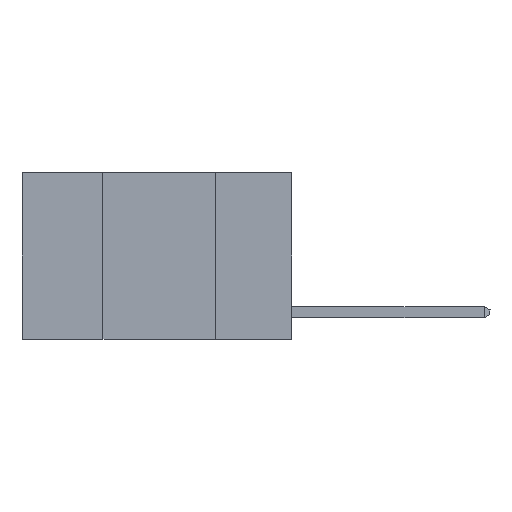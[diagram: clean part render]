
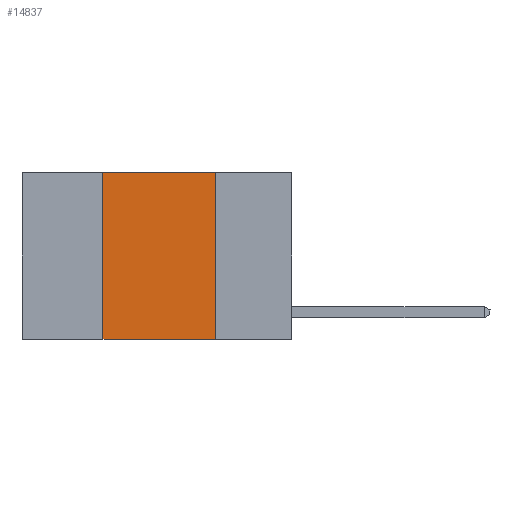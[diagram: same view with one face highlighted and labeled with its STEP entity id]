
A CAD part, left-side view. The second image highlights one B-rep face of the part: STEP entity #14837.
In plain terms, the highlighted planar face has unit normal (-1, 0, 0).
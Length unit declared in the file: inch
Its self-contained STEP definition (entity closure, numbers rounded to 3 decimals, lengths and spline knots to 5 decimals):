
#48 = CARTESIAN_POINT ( 'NONE',  ( 0., 0.42, 0. ) ) ;
#81 = ORIENTED_EDGE ( 'NONE', *, *, #13003, .F. ) ;
#543 = VECTOR ( 'NONE', #5132, 39.37008 ) ;
#2588 = DIRECTION ( 'NONE',  ( 0., -1., 0. ) ) ;
#3650 = DIRECTION ( 'NONE',  ( 0., 0., 1. ) ) ;
#3873 = ORIENTED_EDGE ( 'NONE', *, *, #11862, .F. ) ;
#3981 = CARTESIAN_POINT ( 'NONE',  ( 0., 0.6, 0. ) ) ;
#4129 = CARTESIAN_POINT ( 'NONE',  ( 0., 0.17, -0.37 ) ) ;
#4639 = ORIENTED_EDGE ( 'NONE', *, *, #11732, .T. ) ;
#4916 = PLANE ( 'NONE',  #13979 ) ;
#5132 = DIRECTION ( 'NONE',  ( 0., -1., 0. ) ) ;
#5195 = CARTESIAN_POINT ( 'NONE',  ( 0., 0.17, 0. ) ) ;
#6802 = DIRECTION ( 'NONE',  ( 1., 0., 0. ) ) ;
#6878 = VECTOR ( 'NONE', #3650, 39.37008 ) ;
#7377 = VERTEX_POINT ( 'NONE', #5195 ) ;
#7499 = LINE ( 'NONE', #16522, #9215 ) ;
#8285 = DIRECTION ( 'NONE',  ( 0., 0., -1. ) ) ;
#9215 = VECTOR ( 'NONE', #2588, 39.37008 ) ;
#11022 = DIRECTION ( 'NONE',  ( 0., 0., -1. ) ) ;
#11118 = ORIENTED_EDGE ( 'NONE', *, *, #17581, .F. ) ;
#11295 = LINE ( 'NONE', #12270, #12367 ) ;
#11732 = EDGE_CURVE ( 'NONE', #17272, #11993, #13965, .T. ) ;
#11862 = EDGE_CURVE ( 'NONE', #17272, #14872, #15514, .T. ) ;
#11993 = VERTEX_POINT ( 'NONE', #4129 ) ;
#12173 = EDGE_LOOP ( 'NONE', ( #11118, #81, #3873, #4639 ) ) ;
#12270 = CARTESIAN_POINT ( 'NONE',  ( 0., 0.17, 0. ) ) ;
#12367 = VECTOR ( 'NONE', #11022, 39.37008 ) ;
#13003 = EDGE_CURVE ( 'NONE', #14872, #7377, #7499, .T. ) ;
#13965 = LINE ( 'NONE', #16593, #543 ) ;
#13979 = AXIS2_PLACEMENT_3D ( 'NONE', #3981, #6802, #8285 ) ;
#14837 = ADVANCED_FACE ( 'NONE', ( #17774 ), #4916, .F. ) ;
#14872 = VERTEX_POINT ( 'NONE', #16484 ) ;
#15514 = LINE ( 'NONE', #48, #6878 ) ;
#15637 = CARTESIAN_POINT ( 'NONE',  ( 0., 0.42, -0.37 ) ) ;
#16484 = CARTESIAN_POINT ( 'NONE',  ( 0., 0.42, 0. ) ) ;
#16522 = CARTESIAN_POINT ( 'NONE',  ( 0., 0.6, 0. ) ) ;
#16593 = CARTESIAN_POINT ( 'NONE',  ( 0., 0.6, -0.37 ) ) ;
#17272 = VERTEX_POINT ( 'NONE', #15637 ) ;
#17581 = EDGE_CURVE ( 'NONE', #7377, #11993, #11295, .T. ) ;
#17774 = FACE_OUTER_BOUND ( 'NONE', #12173, .T. ) ;
